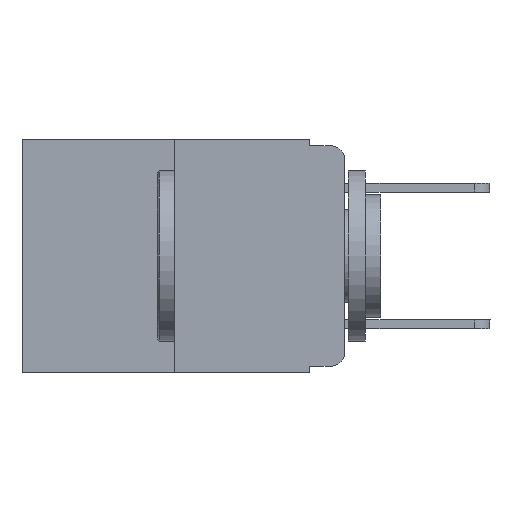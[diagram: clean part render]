
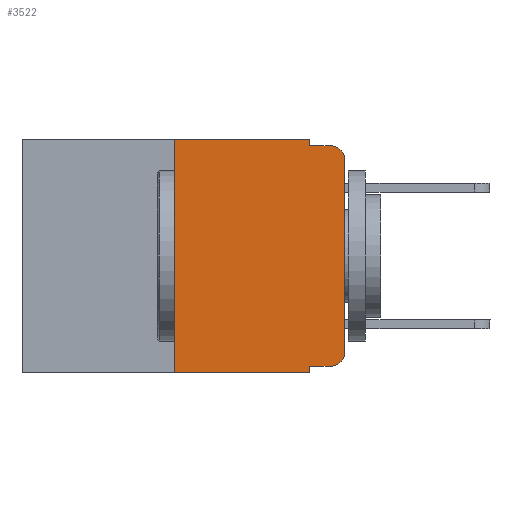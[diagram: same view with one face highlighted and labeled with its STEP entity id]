
A CAD part, left-side view. The second image highlights one B-rep face of the part: STEP entity #3522.
In plain terms, the highlighted planar face has unit normal (-1, 0, 0).
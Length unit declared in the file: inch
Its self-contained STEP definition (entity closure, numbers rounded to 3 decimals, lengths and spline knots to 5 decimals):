
#39 = EDGE_CURVE ( 'NONE', #7376, #2414, #7018, .T. ) ;
#204 = DIRECTION ( 'NONE',  ( 0., 0., -1. ) ) ;
#246 = CIRCLE ( 'NONE', #700, 0.02 ) ;
#380 = VERTEX_POINT ( 'NONE', #4672 ) ;
#523 = VECTOR ( 'NONE', #4773, 39.37008 ) ;
#700 = AXIS2_PLACEMENT_3D ( 'NONE', #3269, #1139, #8250 ) ;
#1139 = DIRECTION ( 'NONE',  ( -1., 0., 0. ) ) ;
#1314 = VECTOR ( 'NONE', #4025, 39.37008 ) ;
#1328 = VERTEX_POINT ( 'NONE', #5822 ) ;
#1332 = LINE ( 'NONE', #7116, #8691 ) ;
#1337 = EDGE_CURVE ( 'NONE', #7308, #2046, #6032, .T. ) ;
#1466 = VERTEX_POINT ( 'NONE', #9691 ) ;
#1817 = EDGE_CURVE ( 'NONE', #6941, #7376, #5162, .T. ) ;
#2046 = VERTEX_POINT ( 'NONE', #3159 ) ;
#2069 = ORIENTED_EDGE ( 'NONE', *, *, #11538, .F. ) ;
#2080 = VECTOR ( 'NONE', #204, 39.37008 ) ;
#2157 = CARTESIAN_POINT ( 'NONE',  ( 0., 0., -0.313 ) ) ;
#2387 = ORIENTED_EDGE ( 'NONE', *, *, #4445, .F. ) ;
#2414 = VERTEX_POINT ( 'NONE', #9062 ) ;
#2606 = ORIENTED_EDGE ( 'NONE', *, *, #8766, .T. ) ;
#2630 = CARTESIAN_POINT ( 'NONE',  ( 0., 0.25, -0.343 ) ) ;
#2696 = PLANE ( 'NONE',  #10133 ) ;
#2819 = CARTESIAN_POINT ( 'NONE',  ( 0., 0.051, -0.01 ) ) ;
#2894 = DIRECTION ( 'NONE',  ( 0., 0., -1. ) ) ;
#3159 = CARTESIAN_POINT ( 'NONE',  ( 0., 0., -0.03 ) ) ;
#3163 = LINE ( 'NONE', #8666, #4255 ) ;
#3269 = CARTESIAN_POINT ( 'NONE',  ( 0., 0.02, -0.03 ) ) ;
#3522 = ADVANCED_FACE ( 'NONE', ( #6701 ), #2696, .F. ) ;
#3641 = ORIENTED_EDGE ( 'NONE', *, *, #7778, .T. ) ;
#3935 = DIRECTION ( 'NONE',  ( 0., -1., 0. ) ) ;
#4009 = CARTESIAN_POINT ( 'NONE',  ( 0., 0.473, -0.343 ) ) ;
#4025 = DIRECTION ( 'NONE',  ( 0., 0., 1. ) ) ;
#4133 = CARTESIAN_POINT ( 'NONE',  ( 0., 0., 0. ) ) ;
#4239 = ORIENTED_EDGE ( 'NONE', *, *, #1337, .T. ) ;
#4255 = VECTOR ( 'NONE', #10360, 39.37008 ) ;
#4409 = DIRECTION ( 'NONE',  ( 1., 0., 0. ) ) ;
#4445 = EDGE_CURVE ( 'NONE', #6892, #6941, #3163, .T. ) ;
#4572 = DIRECTION ( 'NONE',  ( 0., 0., -1. ) ) ;
#4672 = CARTESIAN_POINT ( 'NONE',  ( 0., 0.02, -0.333 ) ) ;
#4773 = DIRECTION ( 'NONE',  ( 0., -1., 0. ) ) ;
#4981 = DIRECTION ( 'NONE',  ( 0., -1., 0. ) ) ;
#5153 = AXIS2_PLACEMENT_3D ( 'NONE', #8204, #5542, #2894 ) ;
#5162 = LINE ( 'NONE', #7336, #8661 ) ;
#5256 = LINE ( 'NONE', #6491, #2080 ) ;
#5542 = DIRECTION ( 'NONE',  ( -1., 0., 0. ) ) ;
#5822 = CARTESIAN_POINT ( 'NONE',  ( 0., 0.051, -0.343 ) ) ;
#6032 = LINE ( 'NONE', #4133, #1314 ) ;
#6056 = VECTOR ( 'NONE', #3935, 39.37008 ) ;
#6113 = CARTESIAN_POINT ( 'NONE',  ( 0., 0.473, 0. ) ) ;
#6372 = ORIENTED_EDGE ( 'NONE', *, *, #9208, .T. ) ;
#6491 = CARTESIAN_POINT ( 'NONE',  ( 0., 0.051, 0. ) ) ;
#6537 = EDGE_LOOP ( 'NONE', ( #4239, #2606, #11479, #9543, #2387, #2069, #11302, #8736, #6372, #3641 ) ) ;
#6701 = FACE_OUTER_BOUND ( 'NONE', #6537, .T. ) ;
#6892 = VERTEX_POINT ( 'NONE', #7686 ) ;
#6941 = VERTEX_POINT ( 'NONE', #10604 ) ;
#6949 = VERTEX_POINT ( 'NONE', #2630 ) ;
#7018 = LINE ( 'NONE', #7775, #8128 ) ;
#7042 = DIRECTION ( 'NONE',  ( 0., 0., 1. ) ) ;
#7116 = CARTESIAN_POINT ( 'NONE',  ( 0., 0.25, 0. ) ) ;
#7216 = LINE ( 'NONE', #8374, #523 ) ;
#7308 = VERTEX_POINT ( 'NONE', #2157 ) ;
#7336 = CARTESIAN_POINT ( 'NONE',  ( 0., 0.051, 0. ) ) ;
#7376 = VERTEX_POINT ( 'NONE', #2819 ) ;
#7686 = CARTESIAN_POINT ( 'NONE',  ( 0., 0.25, 0. ) ) ;
#7775 = CARTESIAN_POINT ( 'NONE',  ( 0., 0.051, -0.01 ) ) ;
#7778 = EDGE_CURVE ( 'NONE', #380, #7308, #9898, .T. ) ;
#8128 = VECTOR ( 'NONE', #4981, 39.37008 ) ;
#8204 = CARTESIAN_POINT ( 'NONE',  ( 0., 0.02, -0.313 ) ) ;
#8250 = DIRECTION ( 'NONE',  ( 0., 0., -1. ) ) ;
#8374 = CARTESIAN_POINT ( 'NONE',  ( 0., 0.051, -0.333 ) ) ;
#8517 = EDGE_CURVE ( 'NONE', #1466, #1328, #5256, .T. ) ;
#8661 = VECTOR ( 'NONE', #4572, 39.37008 ) ;
#8666 = CARTESIAN_POINT ( 'NONE',  ( 0., 0.473, 0. ) ) ;
#8691 = VECTOR ( 'NONE', #7042, 39.37008 ) ;
#8736 = ORIENTED_EDGE ( 'NONE', *, *, #8517, .F. ) ;
#8766 = EDGE_CURVE ( 'NONE', #2046, #2414, #246, .T. ) ;
#9062 = CARTESIAN_POINT ( 'NONE',  ( 0., 0.02, -0.01 ) ) ;
#9208 = EDGE_CURVE ( 'NONE', #1466, #380, #7216, .T. ) ;
#9543 = ORIENTED_EDGE ( 'NONE', *, *, #1817, .F. ) ;
#9691 = CARTESIAN_POINT ( 'NONE',  ( 0., 0.051, -0.333 ) ) ;
#9898 = CIRCLE ( 'NONE', #5153, 0.02 ) ;
#10133 = AXIS2_PLACEMENT_3D ( 'NONE', #6113, #4409, #11524 ) ;
#10360 = DIRECTION ( 'NONE',  ( 0., -1., 0. ) ) ;
#10604 = CARTESIAN_POINT ( 'NONE',  ( 0., 0.051, 0. ) ) ;
#10651 = EDGE_CURVE ( 'NONE', #6949, #1328, #11375, .T. ) ;
#11302 = ORIENTED_EDGE ( 'NONE', *, *, #10651, .T. ) ;
#11375 = LINE ( 'NONE', #4009, #6056 ) ;
#11479 = ORIENTED_EDGE ( 'NONE', *, *, #39, .F. ) ;
#11524 = DIRECTION ( 'NONE',  ( 0., 0., -1. ) ) ;
#11538 = EDGE_CURVE ( 'NONE', #6949, #6892, #1332, .T. ) ;
